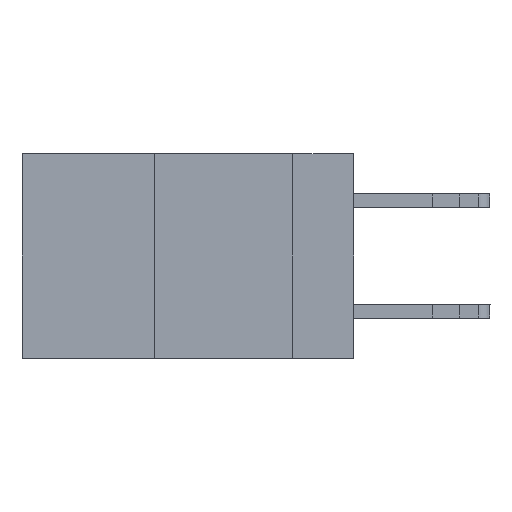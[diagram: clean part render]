
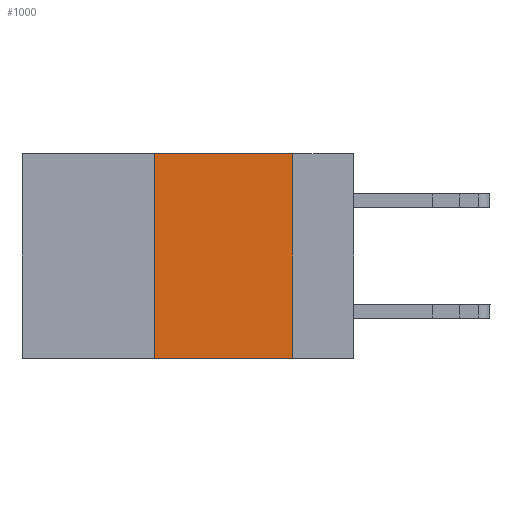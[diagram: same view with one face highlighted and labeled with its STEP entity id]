
A CAD part, left-side view. The second image highlights one B-rep face of the part: STEP entity #1000.
In plain terms, the highlighted planar face has unit normal (-1, 0, 0).
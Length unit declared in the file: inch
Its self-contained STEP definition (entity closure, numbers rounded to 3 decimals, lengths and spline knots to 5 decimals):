
#283 = VERTEX_POINT ( 'NONE', #14097 ) ;
#994 = ORIENTED_EDGE ( 'NONE', *, *, #9189, .F. ) ;
#1000 = ADVANCED_FACE ( 'NONE', ( #18563 ), #18751, .F. ) ;
#1317 = ORIENTED_EDGE ( 'NONE', *, *, #9976, .F. ) ;
#2407 = CARTESIAN_POINT ( 'NONE',  ( 0., 0.36, 0. ) ) ;
#3277 = CARTESIAN_POINT ( 'NONE',  ( 0., 0.6, 0. ) ) ;
#3347 = VECTOR ( 'NONE', #5056, 39.37008 ) ;
#3374 = DIRECTION ( 'NONE',  ( 1., 0., 0. ) ) ;
#4199 = DIRECTION ( 'NONE',  ( 0., 0., -1. ) ) ;
#4355 = VECTOR ( 'NONE', #4199, 39.37008 ) ;
#4769 = VERTEX_POINT ( 'NONE', #9439 ) ;
#4985 = DIRECTION ( 'NONE',  ( 0., 0., -1. ) ) ;
#5056 = DIRECTION ( 'NONE',  ( 0., -1., 0. ) ) ;
#5445 = CARTESIAN_POINT ( 'NONE',  ( 0., 0.6, -0.37 ) ) ;
#5961 = VERTEX_POINT ( 'NONE', #12853 ) ;
#6104 = CARTESIAN_POINT ( 'NONE',  ( 0., 0.6, 0. ) ) ;
#6150 = EDGE_CURVE ( 'NONE', #17553, #5961, #11942, .T. ) ;
#6324 = AXIS2_PLACEMENT_3D ( 'NONE', #3277, #3374, #4985 ) ;
#6577 = VECTOR ( 'NONE', #8771, 39.37008 ) ;
#6892 = ORIENTED_EDGE ( 'NONE', *, *, #9621, .T. ) ;
#8771 = DIRECTION ( 'NONE',  ( 0., -1., 0. ) ) ;
#9189 = EDGE_CURVE ( 'NONE', #4769, #283, #17963, .T. ) ;
#9439 = CARTESIAN_POINT ( 'NONE',  ( 0., 0.11, 0. ) ) ;
#9621 = EDGE_CURVE ( 'NONE', #17553, #283, #10014, .T. ) ;
#9976 = EDGE_CURVE ( 'NONE', #5961, #4769, #18161, .T. ) ;
#10014 = LINE ( 'NONE', #5445, #3347 ) ;
#10569 = CARTESIAN_POINT ( 'NONE',  ( 0., 0.11, 0. ) ) ;
#11835 = ORIENTED_EDGE ( 'NONE', *, *, #6150, .F. ) ;
#11942 = LINE ( 'NONE', #2407, #15945 ) ;
#12853 = CARTESIAN_POINT ( 'NONE',  ( 0., 0.36, 0. ) ) ;
#14097 = CARTESIAN_POINT ( 'NONE',  ( 0., 0.11, -0.37 ) ) ;
#14701 = DIRECTION ( 'NONE',  ( 0., 0., 1. ) ) ;
#14719 = CARTESIAN_POINT ( 'NONE',  ( 0., 0.36, -0.37 ) ) ;
#15945 = VECTOR ( 'NONE', #14701, 39.37008 ) ;
#17046 = EDGE_LOOP ( 'NONE', ( #994, #1317, #11835, #6892 ) ) ;
#17553 = VERTEX_POINT ( 'NONE', #14719 ) ;
#17963 = LINE ( 'NONE', #10569, #4355 ) ;
#18161 = LINE ( 'NONE', #6104, #6577 ) ;
#18563 = FACE_OUTER_BOUND ( 'NONE', #17046, .T. ) ;
#18751 = PLANE ( 'NONE',  #6324 ) ;
